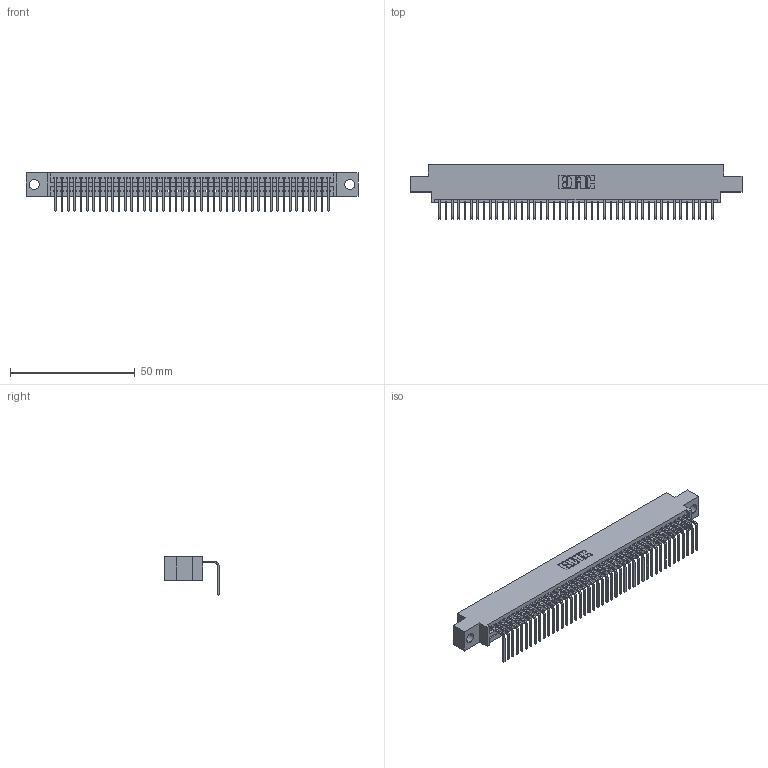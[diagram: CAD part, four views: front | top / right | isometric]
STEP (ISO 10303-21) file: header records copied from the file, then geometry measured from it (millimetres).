
FILE_DESCRIPTION (( 'STEP AP203' ), '1' );
FILE_NAME ('345-044-558-604.STEP', '2021-06-09T16:51:32', ( '' ), ( '' ), 'SwSTEP 2.0', 'SolidWorks 2020', '' );
FILE_SCHEMA (( 'CONFIG_CONTROL_DESIGN' ));
Length unit declared in the file: inch
Products named in the file (3): 345 Part_0.170 Offset - 0.156 Dia-TI; 345-044-558-604; 345-292-001_558 Tail - 2
Assembly tree (45 placements, depth 2):
  345-044-558-604
    345 Part_0.170 Offset - 0.156 Dia-TI
    345-292-001_558 Tail - 2  x44
Bounding box: 132.97 x 21.83 x 15.37 mm (x, y, z)
Volume: 12573.2 mm3; surface area: 17566.2 mm2
Topology: 45 solids, 45 shells, 2784 faces, 8397 edges, 5538 vertices
Faces by surface type: plane 1946, cylinder 838
Entity records: 33481 total; most frequent: CARTESIAN_POINT 5810, ORIENTED_EDGE 5786, DIRECTION 5069, EDGE_CURVE 2893, LINE 2585, VECTOR 2585, VERTEX_POINT 1926, AXIS2_PLACEMENT_3D 1242
